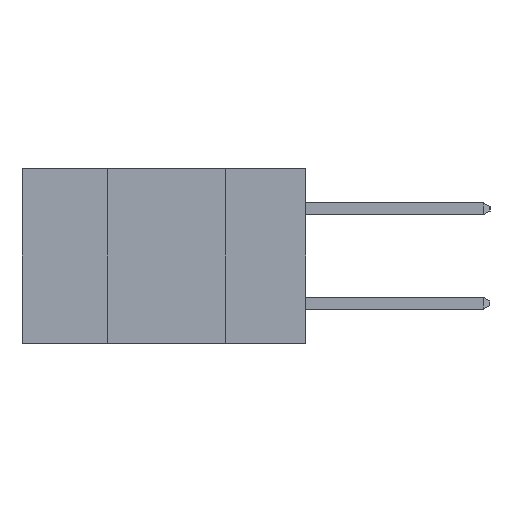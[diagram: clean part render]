
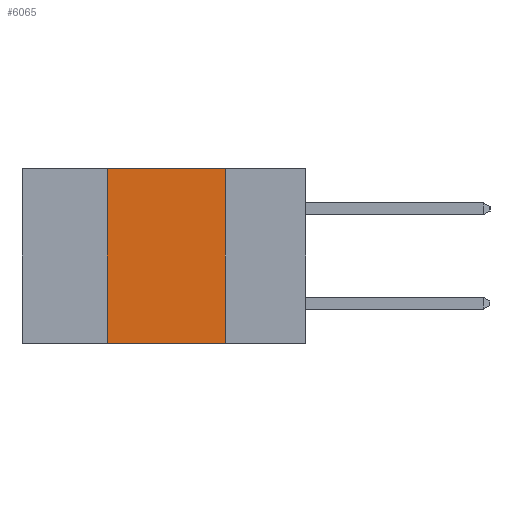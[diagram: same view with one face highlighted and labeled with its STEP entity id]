
A CAD part, left-side view. The second image highlights one B-rep face of the part: STEP entity #6065.
In plain terms, the highlighted planar face has unit normal (-1, 0, 0).
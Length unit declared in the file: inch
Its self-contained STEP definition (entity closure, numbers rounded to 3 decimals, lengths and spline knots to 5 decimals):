
#179 = CARTESIAN_POINT ( 'NONE',  ( 0., 0.17, -0.37 ) ) ;
#513 = LINE ( 'NONE', #1418, #6533 ) ;
#1418 = CARTESIAN_POINT ( 'NONE',  ( 0., 0.6, 0. ) ) ;
#1475 = LINE ( 'NONE', #8371, #10166 ) ;
#2210 = DIRECTION ( 'NONE',  ( 0., -1., 0. ) ) ;
#2299 = DIRECTION ( 'NONE',  ( 0., -1., 0. ) ) ;
#2536 = CARTESIAN_POINT ( 'NONE',  ( 0., 0.17, 0. ) ) ;
#2936 = LINE ( 'NONE', #7042, #6147 ) ;
#3014 = EDGE_CURVE ( 'NONE', #12728, #5056, #2936, .T. ) ;
#3392 = VERTEX_POINT ( 'NONE', #2536 ) ;
#3654 = CARTESIAN_POINT ( 'NONE',  ( 0., 0.42, 0. ) ) ;
#3662 = EDGE_CURVE ( 'NONE', #5211, #3392, #513, .T. ) ;
#4260 = ORIENTED_EDGE ( 'NONE', *, *, #3014, .T. ) ;
#4841 = FACE_OUTER_BOUND ( 'NONE', #11185, .T. ) ;
#5035 = CARTESIAN_POINT ( 'NONE',  ( 0., 0.6, 0. ) ) ;
#5056 = VERTEX_POINT ( 'NONE', #179 ) ;
#5211 = VERTEX_POINT ( 'NONE', #11835 ) ;
#6065 = ADVANCED_FACE ( 'NONE', ( #4841 ), #8099, .F. ) ;
#6147 = VECTOR ( 'NONE', #2299, 39.37008 ) ;
#6533 = VECTOR ( 'NONE', #2210, 39.37008 ) ;
#6808 = ORIENTED_EDGE ( 'NONE', *, *, #3662, .F. ) ;
#7042 = CARTESIAN_POINT ( 'NONE',  ( 0., 0.6, -0.37 ) ) ;
#7636 = LINE ( 'NONE', #3654, #10722 ) ;
#8099 = PLANE ( 'NONE',  #8739 ) ;
#8251 = CARTESIAN_POINT ( 'NONE',  ( 0., 0.42, -0.37 ) ) ;
#8371 = CARTESIAN_POINT ( 'NONE',  ( 0., 0.17, 0. ) ) ;
#8390 = DIRECTION ( 'NONE',  ( 0., 0., 1. ) ) ;
#8739 = AXIS2_PLACEMENT_3D ( 'NONE', #5035, #10137, #12678 ) ;
#10100 = ORIENTED_EDGE ( 'NONE', *, *, #11431, .F. ) ;
#10137 = DIRECTION ( 'NONE',  ( 1., 0., 0. ) ) ;
#10166 = VECTOR ( 'NONE', #11919, 39.37008 ) ;
#10722 = VECTOR ( 'NONE', #8390, 39.37008 ) ;
#11185 = EDGE_LOOP ( 'NONE', ( #14162, #6808, #10100, #4260 ) ) ;
#11431 = EDGE_CURVE ( 'NONE', #12728, #5211, #7636, .T. ) ;
#11835 = CARTESIAN_POINT ( 'NONE',  ( 0., 0.42, 0. ) ) ;
#11919 = DIRECTION ( 'NONE',  ( 0., 0., -1. ) ) ;
#12129 = EDGE_CURVE ( 'NONE', #3392, #5056, #1475, .T. ) ;
#12678 = DIRECTION ( 'NONE',  ( 0., 0., -1. ) ) ;
#12728 = VERTEX_POINT ( 'NONE', #8251 ) ;
#14162 = ORIENTED_EDGE ( 'NONE', *, *, #12129, .F. ) ;
